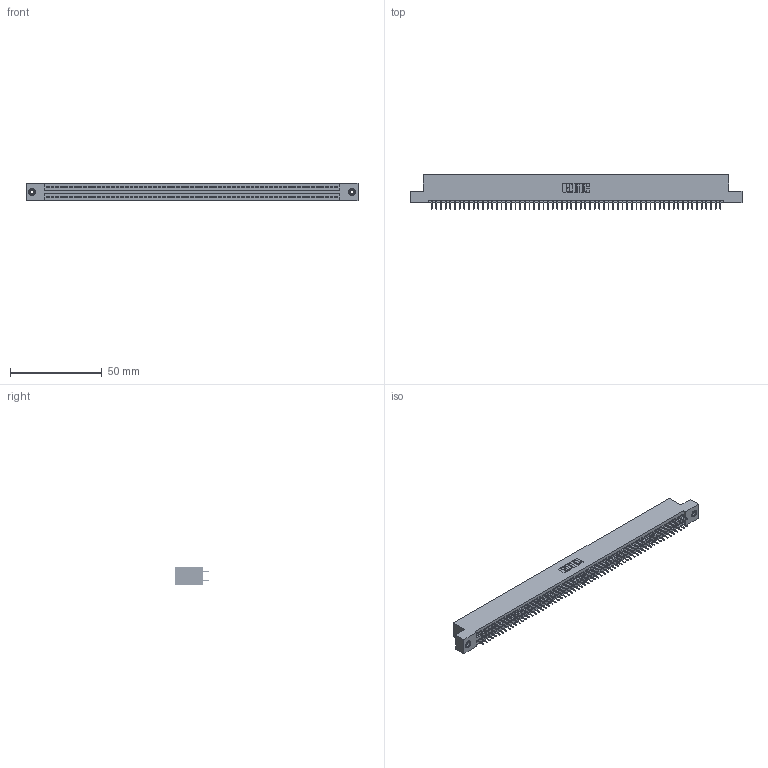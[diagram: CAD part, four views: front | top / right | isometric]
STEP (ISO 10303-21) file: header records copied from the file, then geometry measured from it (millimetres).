
FILE_DESCRIPTION (( 'STEP AP203' ), '1' );
FILE_NAME ('395-126-525-208.STEP', '2020-09-26T00:12:08', ( '' ), ( '' ), 'SwSTEP 2.0', 'SolidWorks 2020', '' );
FILE_SCHEMA (( 'CONFIG_CONTROL_DESIGN' ));
Length unit declared in the file: inch
Products named in the file (4): 345-292-001_345-293-125; 345-250-001_345-250-003-102; 395-126-525-208; 345 Part_Flush Mounting Lugs - 0.156 Dia-TI
Assembly tree (129 placements, depth 2):
  395-126-525-208
    345 Part_Flush Mounting Lugs - 0.156 Dia-TI
    345-292-001_345-293-125  x126
    345-250-001_345-250-003-102  x2
Bounding box: 181.23 x 18.72 x 9.4 mm (x, y, z)
Volume: 17585.8 mm3; surface area: 25789.9 mm2
Topology: 129 solids, 129 shells, 6990 faces, 19755 edges, 12658 vertices
Faces by surface type: plane 5026, cylinder 1948, cone 12, torus 4
Entity records: 47864 total; most frequent: CARTESIAN_POINT 7983, ORIENTED_EDGE 7910, DIRECTION 7041, EDGE_CURVE 3955, LINE 3555, VECTOR 3555, VERTEX_POINT 2628, AXIS2_PLACEMENT_3D 1743
